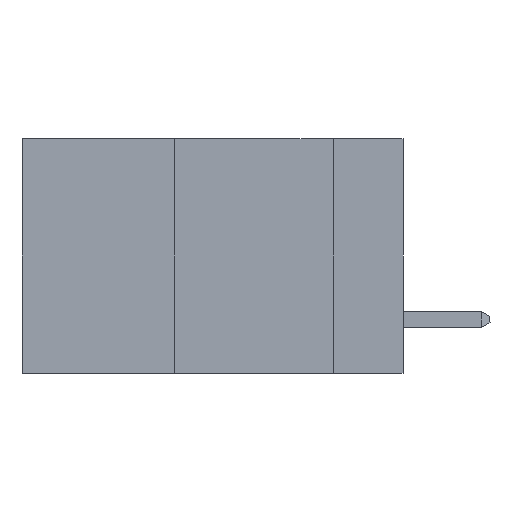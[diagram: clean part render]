
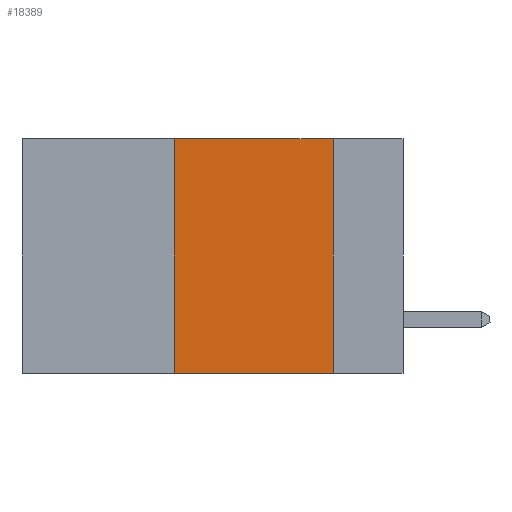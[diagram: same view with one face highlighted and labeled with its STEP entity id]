
A CAD part, left-side view. The second image highlights one B-rep face of the part: STEP entity #18389.
In plain terms, the highlighted planar face has unit normal (-1, 0, 0).
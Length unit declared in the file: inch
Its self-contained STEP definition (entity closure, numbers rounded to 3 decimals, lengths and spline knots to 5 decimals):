
#1045 = PLANE ( 'NONE',  #25786 ) ;
#1115 = DIRECTION ( 'NONE',  ( 0., 0., 1. ) ) ;
#1860 = LINE ( 'NONE', #5536, #8222 ) ;
#3543 = DIRECTION ( 'NONE',  ( 1., 0., 0. ) ) ;
#3669 = EDGE_CURVE ( 'NONE', #9100, #23692, #30004, .T. ) ;
#5252 = VECTOR ( 'NONE', #9708, 39.37008 ) ;
#5536 = CARTESIAN_POINT ( 'NONE',  ( 0., 0.6, 0. ) ) ;
#6098 = ORIENTED_EDGE ( 'NONE', *, *, #29391, .T. ) ;
#7103 = CARTESIAN_POINT ( 'NONE',  ( 0., 0.11, 0. ) ) ;
#7884 = ORIENTED_EDGE ( 'NONE', *, *, #28885, .F. ) ;
#8045 = CARTESIAN_POINT ( 'NONE',  ( 0., 0.36, 0. ) ) ;
#8075 = VECTOR ( 'NONE', #10755, 39.37008 ) ;
#8222 = VECTOR ( 'NONE', #10215, 39.37008 ) ;
#8403 = VERTEX_POINT ( 'NONE', #16944 ) ;
#9100 = VERTEX_POINT ( 'NONE', #26142 ) ;
#9708 = DIRECTION ( 'NONE',  ( 0., -1., 0. ) ) ;
#10215 = DIRECTION ( 'NONE',  ( 0., -1., 0. ) ) ;
#10558 = CARTESIAN_POINT ( 'NONE',  ( 0., 0.36, 0. ) ) ;
#10755 = DIRECTION ( 'NONE',  ( 0., 0., -1. ) ) ;
#12925 = FACE_OUTER_BOUND ( 'NONE', #19348, .T. ) ;
#14128 = ORIENTED_EDGE ( 'NONE', *, *, #3669, .F. ) ;
#16944 = CARTESIAN_POINT ( 'NONE',  ( 0., 0.11, -0.37 ) ) ;
#17659 = CARTESIAN_POINT ( 'NONE',  ( 0., 0.6, 0. ) ) ;
#18389 = ADVANCED_FACE ( 'NONE', ( #12925 ), #1045, .F. ) ;
#19348 = EDGE_LOOP ( 'NONE', ( #22253, #7884, #14128, #6098 ) ) ;
#19892 = LINE ( 'NONE', #24896, #8075 ) ;
#20045 = DIRECTION ( 'NONE',  ( 0., 0., -1. ) ) ;
#22253 = ORIENTED_EDGE ( 'NONE', *, *, #25140, .F. ) ;
#23271 = LINE ( 'NONE', #23824, #5252 ) ;
#23692 = VERTEX_POINT ( 'NONE', #8045 ) ;
#23824 = CARTESIAN_POINT ( 'NONE',  ( 0., 0.6, -0.37 ) ) ;
#23839 = VECTOR ( 'NONE', #1115, 39.37008 ) ;
#24896 = CARTESIAN_POINT ( 'NONE',  ( 0., 0.11, 0. ) ) ;
#25140 = EDGE_CURVE ( 'NONE', #26723, #8403, #19892, .T. ) ;
#25786 = AXIS2_PLACEMENT_3D ( 'NONE', #17659, #3543, #20045 ) ;
#26142 = CARTESIAN_POINT ( 'NONE',  ( 0., 0.36, -0.37 ) ) ;
#26723 = VERTEX_POINT ( 'NONE', #7103 ) ;
#28885 = EDGE_CURVE ( 'NONE', #23692, #26723, #1860, .T. ) ;
#29391 = EDGE_CURVE ( 'NONE', #9100, #8403, #23271, .T. ) ;
#30004 = LINE ( 'NONE', #10558, #23839 ) ;
